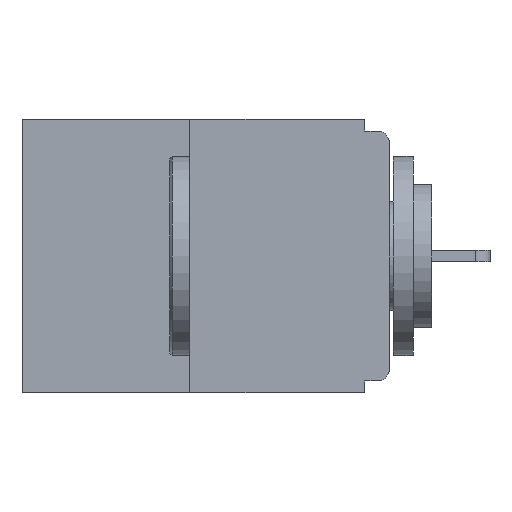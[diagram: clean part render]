
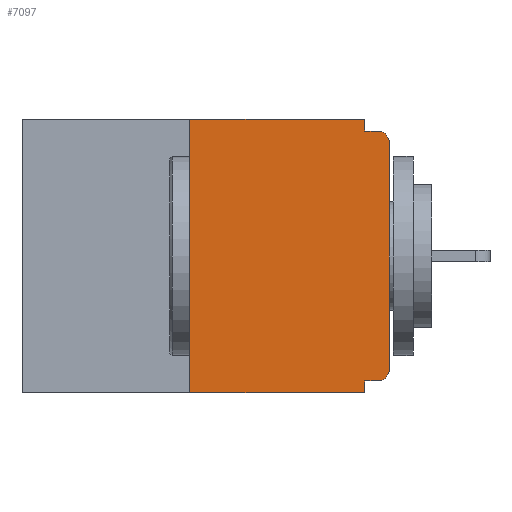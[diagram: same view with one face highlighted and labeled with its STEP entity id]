
A CAD part, left-side view. The second image highlights one B-rep face of the part: STEP entity #7097.
In plain terms, the highlighted planar face has unit normal (-1, 0, 0).
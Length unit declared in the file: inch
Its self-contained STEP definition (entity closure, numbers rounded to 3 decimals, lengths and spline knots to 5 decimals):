
#147 = VECTOR ( 'NONE', #9609, 39.37008 ) ;
#181 = LINE ( 'NONE', #9538, #9487 ) ;
#247 = ORIENTED_EDGE ( 'NONE', *, *, #5061, .T. ) ;
#446 = CARTESIAN_POINT ( 'NONE',  ( 0., 0.031, -0.015 ) ) ;
#633 = ORIENTED_EDGE ( 'NONE', *, *, #4269, .F. ) ;
#948 = VERTEX_POINT ( 'NONE', #974 ) ;
#974 = CARTESIAN_POINT ( 'NONE',  ( 0., 0.25, -0.343 ) ) ;
#1175 = VERTEX_POINT ( 'NONE', #5753 ) ;
#1619 = CARTESIAN_POINT ( 'NONE',  ( 0., 0.031, 0. ) ) ;
#1731 = EDGE_LOOP ( 'NONE', ( #5637, #12224, #247, #633, #7496, #7873, #1825, #11330, #5451, #8617 ) ) ;
#1825 = ORIENTED_EDGE ( 'NONE', *, *, #8181, .T. ) ;
#1827 = LINE ( 'NONE', #11467, #7876 ) ;
#1981 = VECTOR ( 'NONE', #2771, 39.37008 ) ;
#2141 = VECTOR ( 'NONE', #5179, 39.37008 ) ;
#2227 = CARTESIAN_POINT ( 'NONE',  ( 0., 0., 0. ) ) ;
#2771 = DIRECTION ( 'NONE',  ( 0., 0., -1. ) ) ;
#2840 = VERTEX_POINT ( 'NONE', #8618 ) ;
#3439 = CIRCLE ( 'NONE', #5848, 0.015 ) ;
#3458 = EDGE_CURVE ( 'NONE', #14369, #12040, #11478, .T. ) ;
#3463 = DIRECTION ( 'NONE',  ( 0., 0., 1. ) ) ;
#3569 = PLANE ( 'NONE',  #4787 ) ;
#4241 = DIRECTION ( 'NONE',  ( 0., 0., -1. ) ) ;
#4269 = EDGE_CURVE ( 'NONE', #12055, #1175, #181, .T. ) ;
#4434 = DIRECTION ( 'NONE',  ( 1., 0., 0. ) ) ;
#4607 = CIRCLE ( 'NONE', #15230, 0.015 ) ;
#4787 = AXIS2_PLACEMENT_3D ( 'NONE', #11138, #4434, #4241 ) ;
#4963 = CARTESIAN_POINT ( 'NONE',  ( 0., 0.015, -0.015 ) ) ;
#4976 = EDGE_CURVE ( 'NONE', #13342, #12055, #5351, .T. ) ;
#4980 = VECTOR ( 'NONE', #7471, 39.37008 ) ;
#5061 = EDGE_CURVE ( 'NONE', #948, #1175, #12883, .T. ) ;
#5179 = DIRECTION ( 'NONE',  ( 0., -1., 0. ) ) ;
#5268 = VERTEX_POINT ( 'NONE', #11146 ) ;
#5294 = CARTESIAN_POINT ( 'NONE',  ( 0., 0.25, 0. ) ) ;
#5351 = LINE ( 'NONE', #5913, #4980 ) ;
#5365 = LINE ( 'NONE', #13374, #2141 ) ;
#5451 = ORIENTED_EDGE ( 'NONE', *, *, #14606, .F. ) ;
#5484 = DIRECTION ( 'NONE',  ( 0., -1., 0. ) ) ;
#5637 = ORIENTED_EDGE ( 'NONE', *, *, #12523, .F. ) ;
#5753 = CARTESIAN_POINT ( 'NONE',  ( 0., 0.031, -0.343 ) ) ;
#5848 = AXIS2_PLACEMENT_3D ( 'NONE', #13920, #6964, #15028 ) ;
#5913 = CARTESIAN_POINT ( 'NONE',  ( 0., 0., -0.328 ) ) ;
#6354 = CARTESIAN_POINT ( 'NONE',  ( 0., 0.015, -0.313 ) ) ;
#6646 = EDGE_CURVE ( 'NONE', #948, #6771, #1827, .T. ) ;
#6771 = VERTEX_POINT ( 'NONE', #5294 ) ;
#6964 = DIRECTION ( 'NONE',  ( -1., 0., 0. ) ) ;
#7097 = ADVANCED_FACE ( 'NONE', ( #12957 ), #3569, .F. ) ;
#7468 = CARTESIAN_POINT ( 'NONE',  ( 0., 0.031, 0. ) ) ;
#7471 = DIRECTION ( 'NONE',  ( 0., 1., 0. ) ) ;
#7496 = ORIENTED_EDGE ( 'NONE', *, *, #4976, .F. ) ;
#7561 = DIRECTION ( 'NONE',  ( 0., 0., -1. ) ) ;
#7873 = ORIENTED_EDGE ( 'NONE', *, *, #13138, .T. ) ;
#7876 = VECTOR ( 'NONE', #10376, 39.37008 ) ;
#8181 = EDGE_CURVE ( 'NONE', #2840, #5268, #13444, .T. ) ;
#8617 = ORIENTED_EDGE ( 'NONE', *, *, #3458, .F. ) ;
#8618 = CARTESIAN_POINT ( 'NONE',  ( 0., 0., -0.313 ) ) ;
#9487 = VECTOR ( 'NONE', #10664, 39.37008 ) ;
#9538 = CARTESIAN_POINT ( 'NONE',  ( 0., 0.031, -0.343 ) ) ;
#9609 = DIRECTION ( 'NONE',  ( 0., -1., 0. ) ) ;
#10193 = CARTESIAN_POINT ( 'NONE',  ( 0., 0., -0.015 ) ) ;
#10376 = DIRECTION ( 'NONE',  ( 0., 0., 1. ) ) ;
#10406 = VECTOR ( 'NONE', #3463, 39.37008 ) ;
#10664 = DIRECTION ( 'NONE',  ( 0., 0., -1. ) ) ;
#10855 = VERTEX_POINT ( 'NONE', #4963 ) ;
#11138 = CARTESIAN_POINT ( 'NONE',  ( 0., 0.46, 0. ) ) ;
#11146 = CARTESIAN_POINT ( 'NONE',  ( 0., 0., -0.03 ) ) ;
#11330 = ORIENTED_EDGE ( 'NONE', *, *, #11579, .T. ) ;
#11467 = CARTESIAN_POINT ( 'NONE',  ( 0., 0.25, 0. ) ) ;
#11478 = LINE ( 'NONE', #1619, #1981 ) ;
#11579 = EDGE_CURVE ( 'NONE', #5268, #10855, #3439, .T. ) ;
#12040 = VERTEX_POINT ( 'NONE', #446 ) ;
#12055 = VERTEX_POINT ( 'NONE', #13576 ) ;
#12224 = ORIENTED_EDGE ( 'NONE', *, *, #6646, .F. ) ;
#12493 = CARTESIAN_POINT ( 'NONE',  ( 0., 0.015, -0.328 ) ) ;
#12523 = EDGE_CURVE ( 'NONE', #6771, #14369, #5365, .T. ) ;
#12883 = LINE ( 'NONE', #14707, #147 ) ;
#12957 = FACE_OUTER_BOUND ( 'NONE', #1731, .T. ) ;
#13138 = EDGE_CURVE ( 'NONE', #13342, #2840, #4607, .T. ) ;
#13342 = VERTEX_POINT ( 'NONE', #12493 ) ;
#13374 = CARTESIAN_POINT ( 'NONE',  ( 0., 0.46, 0. ) ) ;
#13444 = LINE ( 'NONE', #2227, #10406 ) ;
#13576 = CARTESIAN_POINT ( 'NONE',  ( 0., 0.031, -0.328 ) ) ;
#13725 = LINE ( 'NONE', #10193, #13878 ) ;
#13878 = VECTOR ( 'NONE', #5484, 39.37008 ) ;
#13920 = CARTESIAN_POINT ( 'NONE',  ( 0., 0.015, -0.03 ) ) ;
#14369 = VERTEX_POINT ( 'NONE', #7468 ) ;
#14458 = DIRECTION ( 'NONE',  ( -1., 0., 0. ) ) ;
#14606 = EDGE_CURVE ( 'NONE', #12040, #10855, #13725, .T. ) ;
#14707 = CARTESIAN_POINT ( 'NONE',  ( 0., 0.46, -0.343 ) ) ;
#15028 = DIRECTION ( 'NONE',  ( 0., 0., -1. ) ) ;
#15230 = AXIS2_PLACEMENT_3D ( 'NONE', #6354, #14458, #7561 ) ;
